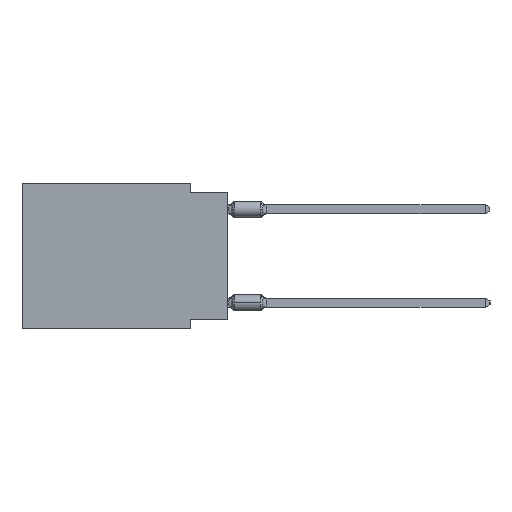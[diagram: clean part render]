
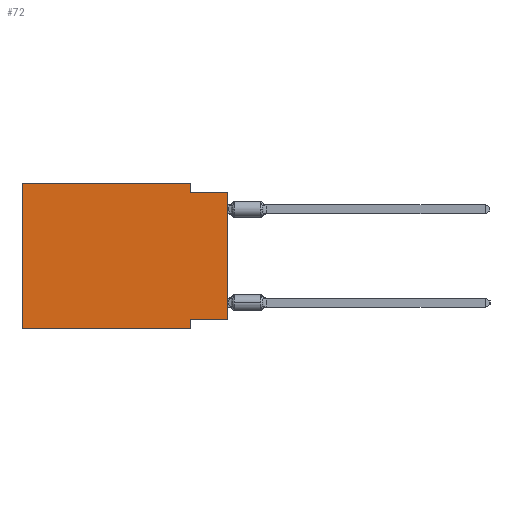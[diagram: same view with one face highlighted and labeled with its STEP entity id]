
A CAD part, left-side view. The second image highlights one B-rep face of the part: STEP entity #72.
In plain terms, the highlighted planar face has unit normal (-1, 0, 0).
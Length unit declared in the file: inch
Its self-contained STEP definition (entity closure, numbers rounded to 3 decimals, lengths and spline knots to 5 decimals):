
#72 = ADVANCED_FACE ( 'NONE', ( #38191 ), #18877, .F. ) ;
#207 = VECTOR ( 'NONE', #46981, 39.37008 ) ;
#685 = LINE ( 'NONE', #10494, #207 ) ;
#1408 = CARTESIAN_POINT ( 'NONE',  ( 0., 0.1, -0.39 ) ) ;
#1869 = CARTESIAN_POINT ( 'NONE',  ( 0., 0., -0.365 ) ) ;
#2043 = VECTOR ( 'NONE', #49306, 39.37008 ) ;
#2951 = ORIENTED_EDGE ( 'NONE', *, *, #9974, .F. ) ;
#3311 = EDGE_CURVE ( 'NONE', #33095, #41823, #13335, .T. ) ;
#4735 = CARTESIAN_POINT ( 'NONE',  ( 0., 0.1, 0. ) ) ;
#5074 = EDGE_LOOP ( 'NONE', ( #44434, #58870, #2951, #32743, #25321, #6905, #20721, #22398 ) ) ;
#5362 = EDGE_CURVE ( 'NONE', #22982, #8389, #53686, .T. ) ;
#6334 = CARTESIAN_POINT ( 'NONE',  ( 0., 0., -0.365 ) ) ;
#6905 = ORIENTED_EDGE ( 'NONE', *, *, #39847, .T. ) ;
#8389 = VERTEX_POINT ( 'NONE', #57830 ) ;
#9974 = EDGE_CURVE ( 'NONE', #41823, #46227, #47657, .T. ) ;
#10494 = CARTESIAN_POINT ( 'NONE',  ( 0., 0.55, 0. ) ) ;
#11406 = VECTOR ( 'NONE', #30676, 39.37008 ) ;
#12664 = LINE ( 'NONE', #31360, #59849 ) ;
#13335 = LINE ( 'NONE', #32336, #46633 ) ;
#14513 = DIRECTION ( 'NONE',  ( 0., 0., -1. ) ) ;
#15436 = DIRECTION ( 'NONE',  ( 0., -1., 0. ) ) ;
#16725 = EDGE_CURVE ( 'NONE', #39650, #33095, #685, .T. ) ;
#16869 = LINE ( 'NONE', #35590, #11406 ) ;
#16991 = AXIS2_PLACEMENT_3D ( 'NONE', #51120, #32995, #23776 ) ;
#17661 = CARTESIAN_POINT ( 'NONE',  ( 0., 0.55, 0. ) ) ;
#17704 = VECTOR ( 'NONE', #14513, 39.37008 ) ;
#18877 = PLANE ( 'NONE',  #16991 ) ;
#20721 = ORIENTED_EDGE ( 'NONE', *, *, #47605, .F. ) ;
#22219 = DIRECTION ( 'NONE',  ( 0., -1., 0. ) ) ;
#22398 = ORIENTED_EDGE ( 'NONE', *, *, #5362, .F. ) ;
#22982 = VERTEX_POINT ( 'NONE', #6334 ) ;
#23415 = VECTOR ( 'NONE', #49080, 39.37008 ) ;
#23776 = DIRECTION ( 'NONE',  ( 0., 0., -1. ) ) ;
#25321 = ORIENTED_EDGE ( 'NONE', *, *, #16725, .F. ) ;
#28271 = CARTESIAN_POINT ( 'NONE',  ( 0., 0.1, -0.025 ) ) ;
#30114 = EDGE_CURVE ( 'NONE', #46227, #41254, #37552, .T. ) ;
#30676 = DIRECTION ( 'NONE',  ( 0., -1., 0. ) ) ;
#31360 = CARTESIAN_POINT ( 'NONE',  ( 0., 0.1, -0.39 ) ) ;
#31452 = CARTESIAN_POINT ( 'NONE',  ( 0., 0.1, 0. ) ) ;
#31686 = EDGE_CURVE ( 'NONE', #22982, #41254, #35779, .T. ) ;
#32336 = CARTESIAN_POINT ( 'NONE',  ( 0., 0.55, 0. ) ) ;
#32743 = ORIENTED_EDGE ( 'NONE', *, *, #3311, .F. ) ;
#32995 = DIRECTION ( 'NONE',  ( 1., 0., 0. ) ) ;
#33095 = VERTEX_POINT ( 'NONE', #17661 ) ;
#35590 = CARTESIAN_POINT ( 'NONE',  ( 0., 0.55, -0.39 ) ) ;
#35779 = LINE ( 'NONE', #58214, #2043 ) ;
#37552 = LINE ( 'NONE', #47049, #42250 ) ;
#38191 = FACE_OUTER_BOUND ( 'NONE', #5074, .T. ) ;
#39650 = VERTEX_POINT ( 'NONE', #42714 ) ;
#39847 = EDGE_CURVE ( 'NONE', #39650, #55759, #16869, .T. ) ;
#40899 = DIRECTION ( 'NONE',  ( 0., 0., -1. ) ) ;
#41254 = VERTEX_POINT ( 'NONE', #53656 ) ;
#41823 = VERTEX_POINT ( 'NONE', #31452 ) ;
#42250 = VECTOR ( 'NONE', #15436, 39.37008 ) ;
#42714 = CARTESIAN_POINT ( 'NONE',  ( 0., 0.55, -0.39 ) ) ;
#44434 = ORIENTED_EDGE ( 'NONE', *, *, #31686, .T. ) ;
#46227 = VERTEX_POINT ( 'NONE', #28271 ) ;
#46633 = VECTOR ( 'NONE', #22219, 39.37008 ) ;
#46981 = DIRECTION ( 'NONE',  ( 0., 0., 1. ) ) ;
#47049 = CARTESIAN_POINT ( 'NONE',  ( 0., 0., -0.025 ) ) ;
#47605 = EDGE_CURVE ( 'NONE', #8389, #55759, #12664, .T. ) ;
#47657 = LINE ( 'NONE', #4735, #17704 ) ;
#49080 = DIRECTION ( 'NONE',  ( 0., 1., 0. ) ) ;
#49306 = DIRECTION ( 'NONE',  ( 0., 0., 1. ) ) ;
#51120 = CARTESIAN_POINT ( 'NONE',  ( 0., 0.55, 0. ) ) ;
#53656 = CARTESIAN_POINT ( 'NONE',  ( 0., 0., -0.025 ) ) ;
#53686 = LINE ( 'NONE', #1869, #23415 ) ;
#55759 = VERTEX_POINT ( 'NONE', #1408 ) ;
#57830 = CARTESIAN_POINT ( 'NONE',  ( 0., 0.1, -0.365 ) ) ;
#58214 = CARTESIAN_POINT ( 'NONE',  ( 0., 0., 0. ) ) ;
#58870 = ORIENTED_EDGE ( 'NONE', *, *, #30114, .F. ) ;
#59849 = VECTOR ( 'NONE', #40899, 39.37008 ) ;
